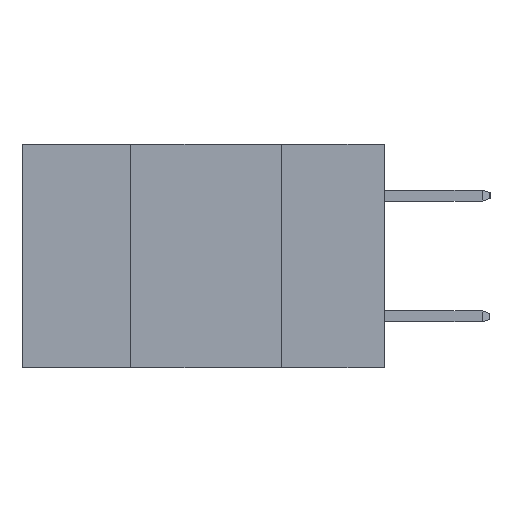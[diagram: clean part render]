
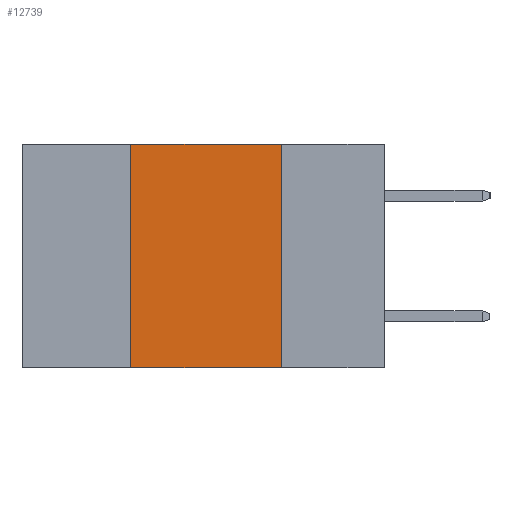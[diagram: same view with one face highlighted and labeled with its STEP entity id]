
A CAD part, left-side view. The second image highlights one B-rep face of the part: STEP entity #12739.
In plain terms, the highlighted planar face has unit normal (-1, 0, 0).
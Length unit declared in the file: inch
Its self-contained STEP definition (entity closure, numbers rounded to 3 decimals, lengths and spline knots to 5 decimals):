
#549 = CARTESIAN_POINT ( 'NONE',  ( 0., 0.6, -0.37 ) ) ;
#610 = DIRECTION ( 'NONE',  ( 0., -1., 0. ) ) ;
#1298 = CARTESIAN_POINT ( 'NONE',  ( 0., 0.17, 0. ) ) ;
#1317 = ORIENTED_EDGE ( 'NONE', *, *, #14179, .F. ) ;
#2048 = VECTOR ( 'NONE', #10613, 39.37008 ) ;
#2062 = AXIS2_PLACEMENT_3D ( 'NONE', #15882, #8022, #17220 ) ;
#2337 = CARTESIAN_POINT ( 'NONE',  ( 0., 0.17, -0.37 ) ) ;
#2650 = DIRECTION ( 'NONE',  ( 0., 0., -1. ) ) ;
#3902 = VECTOR ( 'NONE', #8396, 39.37008 ) ;
#4039 = VECTOR ( 'NONE', #610, 39.37008 ) ;
#5028 = EDGE_CURVE ( 'NONE', #10975, #11059, #7685, .T. ) ;
#6660 = PLANE ( 'NONE',  #2062 ) ;
#7106 = LINE ( 'NONE', #8335, #3902 ) ;
#7299 = ORIENTED_EDGE ( 'NONE', *, *, #12735, .F. ) ;
#7685 = LINE ( 'NONE', #549, #4039 ) ;
#8022 = DIRECTION ( 'NONE',  ( 1., 0., 0. ) ) ;
#8335 = CARTESIAN_POINT ( 'NONE',  ( 0., 0.42, 0. ) ) ;
#8396 = DIRECTION ( 'NONE',  ( 0., 0., 1. ) ) ;
#8809 = VERTEX_POINT ( 'NONE', #16714 ) ;
#8976 = ORIENTED_EDGE ( 'NONE', *, *, #5028, .T. ) ;
#9250 = LINE ( 'NONE', #9299, #2048 ) ;
#9299 = CARTESIAN_POINT ( 'NONE',  ( 0., 0.6, 0. ) ) ;
#10613 = DIRECTION ( 'NONE',  ( 0., -1., 0. ) ) ;
#10965 = VECTOR ( 'NONE', #2650, 39.37008 ) ;
#10975 = VERTEX_POINT ( 'NONE', #16781 ) ;
#11059 = VERTEX_POINT ( 'NONE', #2337 ) ;
#11803 = LINE ( 'NONE', #1298, #10965 ) ;
#12314 = FACE_OUTER_BOUND ( 'NONE', #16423, .T. ) ;
#12735 = EDGE_CURVE ( 'NONE', #14813, #8809, #9250, .T. ) ;
#12739 = ADVANCED_FACE ( 'NONE', ( #12314 ), #6660, .F. ) ;
#13451 = ORIENTED_EDGE ( 'NONE', *, *, #14726, .F. ) ;
#13522 = CARTESIAN_POINT ( 'NONE',  ( 0., 0.42, 0. ) ) ;
#14179 = EDGE_CURVE ( 'NONE', #10975, #14813, #7106, .T. ) ;
#14726 = EDGE_CURVE ( 'NONE', #8809, #11059, #11803, .T. ) ;
#14813 = VERTEX_POINT ( 'NONE', #13522 ) ;
#15882 = CARTESIAN_POINT ( 'NONE',  ( 0., 0.6, 0. ) ) ;
#16423 = EDGE_LOOP ( 'NONE', ( #13451, #7299, #1317, #8976 ) ) ;
#16714 = CARTESIAN_POINT ( 'NONE',  ( 0., 0.17, 0. ) ) ;
#16781 = CARTESIAN_POINT ( 'NONE',  ( 0., 0.42, -0.37 ) ) ;
#17220 = DIRECTION ( 'NONE',  ( 0., 0., -1. ) ) ;
